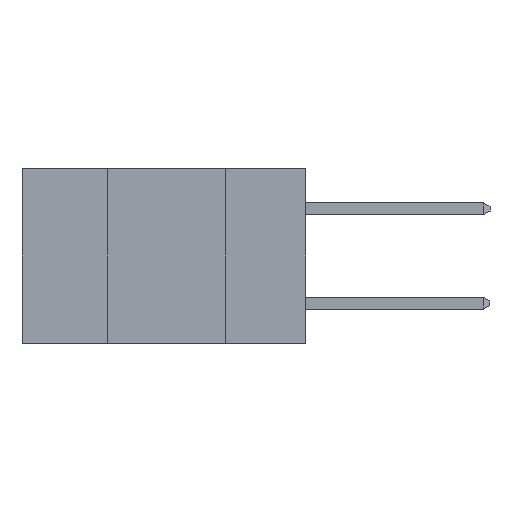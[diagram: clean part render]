
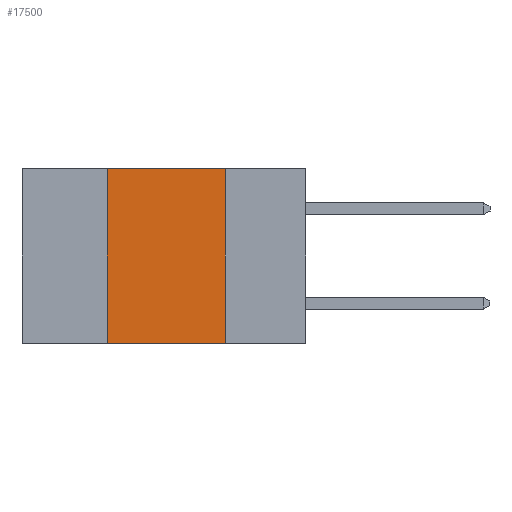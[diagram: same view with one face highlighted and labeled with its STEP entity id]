
A CAD part, left-side view. The second image highlights one B-rep face of the part: STEP entity #17500.
In plain terms, the highlighted planar face has unit normal (-1, 0, 0).
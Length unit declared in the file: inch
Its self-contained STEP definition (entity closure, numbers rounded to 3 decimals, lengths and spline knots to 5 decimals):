
#1187 = EDGE_CURVE ( 'NONE', #8913, #6086, #22482, .T. ) ;
#1809 = CARTESIAN_POINT ( 'NONE',  ( 0., 0.6, 0. ) ) ;
#2831 = CARTESIAN_POINT ( 'NONE',  ( 0., 0.42, 0. ) ) ;
#3215 = CARTESIAN_POINT ( 'NONE',  ( 0., 0.42, 0. ) ) ;
#4031 = DIRECTION ( 'NONE',  ( 0., 0., -1. ) ) ;
#6086 = VERTEX_POINT ( 'NONE', #18338 ) ;
#6719 = EDGE_LOOP ( 'NONE', ( #23993, #25630, #8071, #20894 ) ) ;
#8071 = ORIENTED_EDGE ( 'NONE', *, *, #18946, .F. ) ;
#8254 = CARTESIAN_POINT ( 'NONE',  ( 0., 0.17, -0.37 ) ) ;
#8913 = VERTEX_POINT ( 'NONE', #3215 ) ;
#9312 = CARTESIAN_POINT ( 'NONE',  ( 0., 0.42, -0.37 ) ) ;
#10699 = LINE ( 'NONE', #26734, #21451 ) ;
#12624 = EDGE_CURVE ( 'NONE', #22091, #23165, #10699, .T. ) ;
#12649 = CARTESIAN_POINT ( 'NONE',  ( 0., 0.6, 0. ) ) ;
#13795 = DIRECTION ( 'NONE',  ( 0., -1., 0. ) ) ;
#13959 = FACE_OUTER_BOUND ( 'NONE', #6719, .T. ) ;
#16062 = EDGE_CURVE ( 'NONE', #6086, #23165, #18089, .T. ) ;
#17125 = DIRECTION ( 'NONE',  ( 1., 0., 0. ) ) ;
#17500 = ADVANCED_FACE ( 'NONE', ( #13959 ), #25616, .F. ) ;
#18089 = LINE ( 'NONE', #27287, #22462 ) ;
#18338 = CARTESIAN_POINT ( 'NONE',  ( 0., 0.17, 0. ) ) ;
#18946 = EDGE_CURVE ( 'NONE', #22091, #8913, #21942, .T. ) ;
#20894 = ORIENTED_EDGE ( 'NONE', *, *, #12624, .T. ) ;
#21451 = VECTOR ( 'NONE', #13795, 39.37008 ) ;
#21942 = LINE ( 'NONE', #2831, #22631 ) ;
#22091 = VERTEX_POINT ( 'NONE', #9312 ) ;
#22462 = VECTOR ( 'NONE', #23026, 39.37008 ) ;
#22482 = LINE ( 'NONE', #12649, #26890 ) ;
#22631 = VECTOR ( 'NONE', #24611, 39.37008 ) ;
#23026 = DIRECTION ( 'NONE',  ( 0., 0., -1. ) ) ;
#23165 = VERTEX_POINT ( 'NONE', #8254 ) ;
#23644 = DIRECTION ( 'NONE',  ( 0., -1., 0. ) ) ;
#23993 = ORIENTED_EDGE ( 'NONE', *, *, #16062, .F. ) ;
#24611 = DIRECTION ( 'NONE',  ( 0., 0., 1. ) ) ;
#25616 = PLANE ( 'NONE',  #27198 ) ;
#25630 = ORIENTED_EDGE ( 'NONE', *, *, #1187, .F. ) ;
#26734 = CARTESIAN_POINT ( 'NONE',  ( 0., 0.6, -0.37 ) ) ;
#26890 = VECTOR ( 'NONE', #23644, 39.37008 ) ;
#27198 = AXIS2_PLACEMENT_3D ( 'NONE', #1809, #17125, #4031 ) ;
#27287 = CARTESIAN_POINT ( 'NONE',  ( 0., 0.17, 0. ) ) ;
